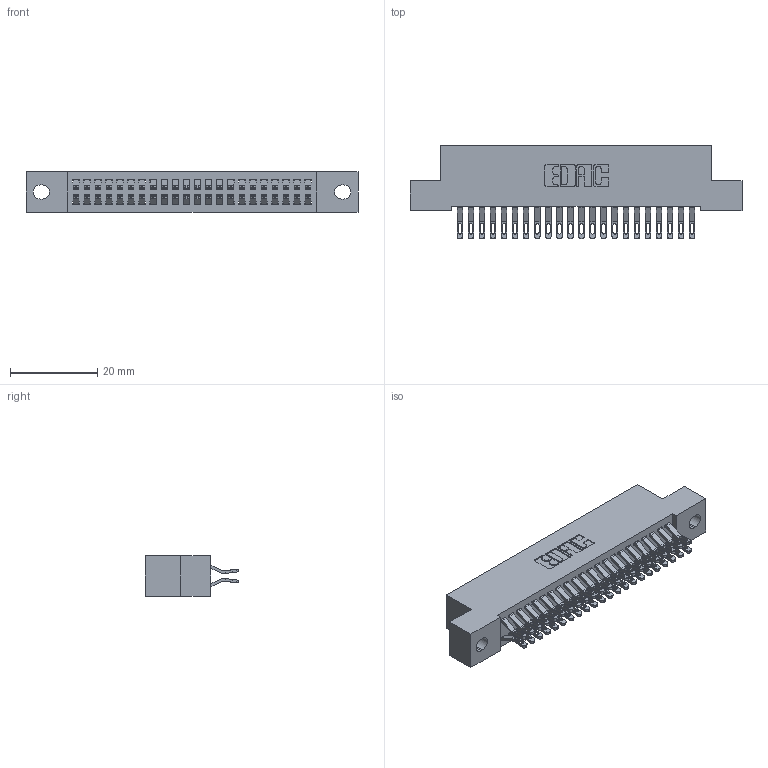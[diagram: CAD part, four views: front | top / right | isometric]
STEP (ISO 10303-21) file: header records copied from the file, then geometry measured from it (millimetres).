
FILE_DESCRIPTION (( 'STEP AP203' ), '1' );
FILE_NAME ('392-044-555-202.STEP', '2018-08-16T15:28:20', ( '' ), ( '' ), 'SwSTEP 2.0', 'SolidWorks 2016', '' );
FILE_SCHEMA (( 'CONFIG_CONTROL_DESIGN' ));
Length unit declared in the file: inch
Products named in the file (3): 342 Part_.128 Slot; 345-292-001_555 Tail; 392-044-555-202
Assembly tree (45 placements, depth 2):
  392-044-555-202
    342 Part_.128 Slot
    345-292-001_555 Tail  x44
Bounding box: 76.2 x 21.47 x 9.4 mm (x, y, z)
Volume: 6822 mm3; surface area: 10796.9 mm2
Topology: 45 solids, 45 shells, 2666 faces, 8363 edges, 5574 vertices
Faces by surface type: plane 1566, cylinder 1100
Entity records: 17069 total; most frequent: CARTESIAN_POINT 2888, ORIENTED_EDGE 2794, DIRECTION 2473, EDGE_CURVE 1397, LINE 1249, VECTOR 1249, VERTEX_POINT 930, AXIS2_PLACEMENT_3D 612
